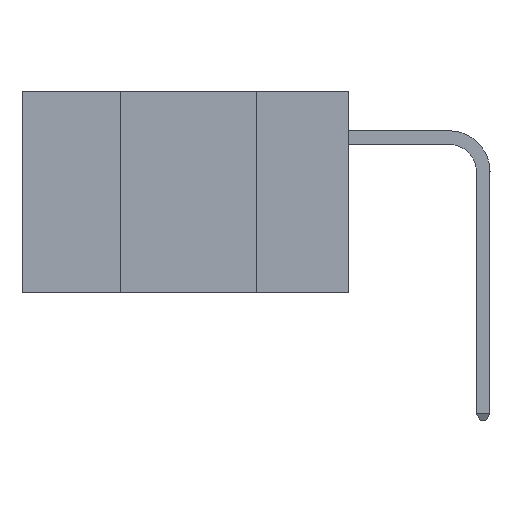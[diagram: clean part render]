
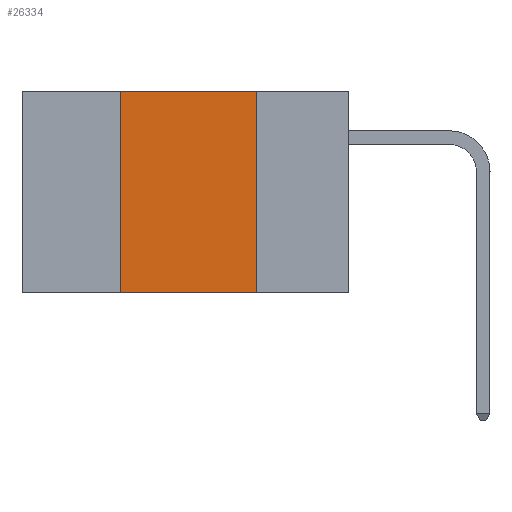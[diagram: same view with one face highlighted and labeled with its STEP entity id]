
A CAD part, left-side view. The second image highlights one B-rep face of the part: STEP entity #26334.
In plain terms, the highlighted planar face has unit normal (-1, 0, 0).
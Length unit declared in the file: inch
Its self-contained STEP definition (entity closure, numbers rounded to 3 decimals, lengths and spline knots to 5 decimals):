
#281 = LINE ( 'NONE', #4868, #14239 ) ;
#895 = CARTESIAN_POINT ( 'NONE',  ( 0., 0.6, -0.37 ) ) ;
#1497 = DIRECTION ( 'NONE',  ( 1., 0., 0. ) ) ;
#3115 = EDGE_LOOP ( 'NONE', ( #23586, #34943, #5518, #30761 ) ) ;
#4868 = CARTESIAN_POINT ( 'NONE',  ( 0., 0.17, 0. ) ) ;
#5518 = ORIENTED_EDGE ( 'NONE', *, *, #8871, .F. ) ;
#6560 = DIRECTION ( 'NONE',  ( 0., -1., 0. ) ) ;
#6731 = EDGE_CURVE ( 'NONE', #35305, #11549, #281, .T. ) ;
#8871 = EDGE_CURVE ( 'NONE', #34185, #20391, #26568, .T. ) ;
#11549 = VERTEX_POINT ( 'NONE', #34133 ) ;
#11817 = VECTOR ( 'NONE', #12652, 39.37008 ) ;
#12033 = VECTOR ( 'NONE', #20422, 39.37008 ) ;
#12652 = DIRECTION ( 'NONE',  ( 0., -1., 0. ) ) ;
#13860 = EDGE_CURVE ( 'NONE', #34185, #11549, #28672, .T. ) ;
#14239 = VECTOR ( 'NONE', #29630, 39.37008 ) ;
#15434 = CARTESIAN_POINT ( 'NONE',  ( 0., 0.17, 0. ) ) ;
#17656 = CARTESIAN_POINT ( 'NONE',  ( 0., 0.42, 0. ) ) ;
#18107 = CARTESIAN_POINT ( 'NONE',  ( 0., 0.6, 0. ) ) ;
#19928 = FACE_OUTER_BOUND ( 'NONE', #3115, .T. ) ;
#19967 = LINE ( 'NONE', #31682, #11817 ) ;
#20391 = VERTEX_POINT ( 'NONE', #33874 ) ;
#20422 = DIRECTION ( 'NONE',  ( 0., 0., 1. ) ) ;
#20880 = DIRECTION ( 'NONE',  ( 0., 0., -1. ) ) ;
#23535 = PLANE ( 'NONE',  #30456 ) ;
#23586 = ORIENTED_EDGE ( 'NONE', *, *, #6731, .F. ) ;
#25727 = EDGE_CURVE ( 'NONE', #20391, #35305, #19967, .T. ) ;
#26334 = ADVANCED_FACE ( 'NONE', ( #19928 ), #23535, .F. ) ;
#26568 = LINE ( 'NONE', #17656, #12033 ) ;
#28672 = LINE ( 'NONE', #895, #34995 ) ;
#29630 = DIRECTION ( 'NONE',  ( 0., 0., -1. ) ) ;
#30456 = AXIS2_PLACEMENT_3D ( 'NONE', #18107, #1497, #20880 ) ;
#30761 = ORIENTED_EDGE ( 'NONE', *, *, #13860, .T. ) ;
#31682 = CARTESIAN_POINT ( 'NONE',  ( 0., 0.6, 0. ) ) ;
#33874 = CARTESIAN_POINT ( 'NONE',  ( 0., 0.42, 0. ) ) ;
#34133 = CARTESIAN_POINT ( 'NONE',  ( 0., 0.17, -0.37 ) ) ;
#34185 = VERTEX_POINT ( 'NONE', #35435 ) ;
#34943 = ORIENTED_EDGE ( 'NONE', *, *, #25727, .F. ) ;
#34995 = VECTOR ( 'NONE', #6560, 39.37008 ) ;
#35305 = VERTEX_POINT ( 'NONE', #15434 ) ;
#35435 = CARTESIAN_POINT ( 'NONE',  ( 0., 0.42, -0.37 ) ) ;
